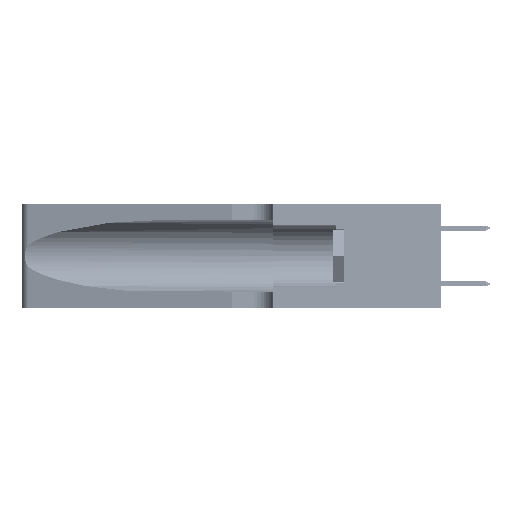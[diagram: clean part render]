
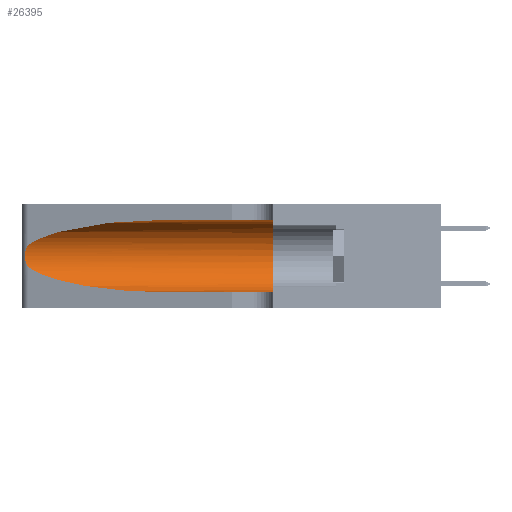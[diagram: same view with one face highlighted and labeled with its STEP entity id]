
A CAD part, left-side view. The second image highlights one B-rep face of the part: STEP entity #26395.
In plain terms, the highlighted cylindrical face has radius 3.308 mm (diameter 6.617 mm), a partial arc.
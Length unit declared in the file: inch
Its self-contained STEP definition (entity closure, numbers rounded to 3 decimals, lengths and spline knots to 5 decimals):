
#160 = CARTESIAN_POINT ( 'NONE',  ( 0.26075, 1.23896, 0.19203 ) ) ;
#484 = CARTESIAN_POINT ( 'NONE',  ( 0.25787, 1.23484, 0.2124 ) ) ;
#584 = VERTEX_POINT ( 'NONE', #38833 ) ;
#1126 = AXIS2_PLACEMENT_3D ( 'NONE', #7412, #33444, #25333 ) ;
#3918 = CARTESIAN_POINT ( 'NONE',  ( 0.25639, 1.23184, 0.21858 ) ) ;
#4160 = CARTESIAN_POINT ( 'NONE',  ( 0.25487, 1.22718, 0.22369 ) ) ;
#6103 = CYLINDRICAL_SURFACE ( 'NONE', #1126, 0.13025 ) ;
#6865 = DIRECTION ( 'NONE',  ( 0., 1., 0. ) ) ;
#7412 = CARTESIAN_POINT ( 'NONE',  ( 0.1305, 1.61858, 0.185 ) ) ;
#7413 = CIRCLE ( 'NONE', #36605, 0.13025 ) ;
#7714 = CARTESIAN_POINT ( 'NONE',  ( 0.18966, 0.96281, 0.31525 ) ) ;
#7722 = EDGE_CURVE ( 'NONE', #584, #17332, #21143, .T. ) ;
#8192 = CARTESIAN_POINT ( 'NONE',  ( 0.1305, 0.72297, 0.31525 ) ) ;
#9548 =( BOUNDED_CURVE ( )  B_SPLINE_CURVE ( 3, ( #43768, #21286, #43301, #39689 ),
 .UNSPECIFIED., .F., .F. ) 
 B_SPLINE_CURVE_WITH_KNOTS ( ( 4, 4 ),
 ( 3.44316, 4.71239 ),
 .UNSPECIFIED. ) 
 CURVE ( )  GEOMETRIC_REPRESENTATION_ITEM ( )  RATIONAL_B_SPLINE_CURVE ( ( 1., 0.87, 0.87, 1. ) ) 
 REPRESENTATION_ITEM ( '' )  );
#9904 = ORIENTED_EDGE ( 'NONE', *, *, #37767, .F. ) ;
#10907 = CARTESIAN_POINT ( 'NONE',  ( 0.25487, 1.22718, 0.14631 ) ) ;
#11216 = EDGE_CURVE ( 'NONE', #584, #25599, #27756, .T. ) ;
#14058 = CARTESIAN_POINT ( 'NONE',  ( 0.1305, 0.72297, 0.05475 ) ) ;
#14663 = ORIENTED_EDGE ( 'NONE', *, *, #36553, .T. ) ;
#15286 = CARTESIAN_POINT ( 'NONE',  ( 0.25487, 1.22718, 0.22369 ) ) ;
#15588 = ORIENTED_EDGE ( 'NONE', *, *, #11216, .T. ) ;
#17234 = EDGE_CURVE ( 'NONE', #25599, #41926, #20280, .T. ) ;
#17332 = VERTEX_POINT ( 'NONE', #23597 ) ;
#20280 = B_SPLINE_CURVE_WITH_KNOTS ( 'NONE', 3,
 ( #15286, #22461, #3918, #484, #44805, #48227, #160, #37453, #22783, #25884, #22613, #26208, #33673, #10907 ),
 .UNSPECIFIED., .F., .F.,
 ( 4, 2, 2, 2, 2, 2, 4 ),
 ( 0., 0.00027, 0.00053, 0.00107, 0.0016, 0.00187, 0.00214 ),
 .UNSPECIFIED. ) ;
#21143 = LINE ( 'NONE', #32674, #31049 ) ;
#21286 = CARTESIAN_POINT ( 'NONE',  ( 0.2373, 1.15595, 0.08982 ) ) ;
#22092 = CARTESIAN_POINT ( 'NONE',  ( 0.1305, 1.61858, 0.05475 ) ) ;
#22461 = CARTESIAN_POINT ( 'NONE',  ( 0.25555, 1.22994, 0.2215 ) ) ;
#22613 = CARTESIAN_POINT ( 'NONE',  ( 0.25789, 1.23486, 0.15765 ) ) ;
#22783 = CARTESIAN_POINT ( 'NONE',  ( 0.26017, 1.23833, 0.17102 ) ) ;
#23597 = CARTESIAN_POINT ( 'NONE',  ( 0.1305, 0.35, 0.31525 ) ) ;
#24653 = FACE_OUTER_BOUND ( 'NONE', #31269, .T. ) ;
#25333 = DIRECTION ( 'NONE',  ( 0., 0., -1. ) ) ;
#25599 = VERTEX_POINT ( 'NONE', #31252 ) ;
#25884 = CARTESIAN_POINT ( 'NONE',  ( 0.25856, 1.23593, 0.16098 ) ) ;
#26208 = CARTESIAN_POINT ( 'NONE',  ( 0.25639, 1.23186, 0.15144 ) ) ;
#26395 = ADVANCED_FACE ( 'NONE', ( #24653 ), #6103, .F. ) ;
#27756 =( BOUNDED_CURVE ( )  B_SPLINE_CURVE ( 3, ( #8192, #7714, #41251, #4160 ),
 .UNSPECIFIED., .F., .F. ) 
 B_SPLINE_CURVE_WITH_KNOTS ( ( 4, 4 ),
 ( 1.5708, 2.84003 ),
 .UNSPECIFIED. ) 
 CURVE ( )  GEOMETRIC_REPRESENTATION_ITEM ( )  RATIONAL_B_SPLINE_CURVE ( ( 1., 0.87, 0.87, 1. ) ) 
 REPRESENTATION_ITEM ( '' )  );
#29281 = DIRECTION ( 'NONE',  ( 0., -1., 0. ) ) ;
#29341 = VERTEX_POINT ( 'NONE', #38858 ) ;
#29375 = VERTEX_POINT ( 'NONE', #14058 ) ;
#31049 = VECTOR ( 'NONE', #47052, 39.37008 ) ;
#31252 = CARTESIAN_POINT ( 'NONE',  ( 0.25487, 1.22718, 0.22369 ) ) ;
#31269 = EDGE_LOOP ( 'NONE', ( #15588, #44479, #36143, #14663, #9904, #44115 ) ) ;
#32674 = CARTESIAN_POINT ( 'NONE',  ( 0.1305, 1.61858, 0.31525 ) ) ;
#33444 = DIRECTION ( 'NONE',  ( 0., -1., 0. ) ) ;
#33673 = CARTESIAN_POINT ( 'NONE',  ( 0.25555, 1.22993, 0.14849 ) ) ;
#35210 = EDGE_CURVE ( 'NONE', #41926, #29375, #9548, .T. ) ;
#36143 = ORIENTED_EDGE ( 'NONE', *, *, #35210, .T. ) ;
#36553 = EDGE_CURVE ( 'NONE', #29375, #29341, #36727, .T. ) ;
#36605 = AXIS2_PLACEMENT_3D ( 'NONE', #48054, #6865, #43981 ) ;
#36727 = LINE ( 'NONE', #22092, #43153 ) ;
#37453 = CARTESIAN_POINT ( 'NONE',  ( 0.26075, 1.23896, 0.178 ) ) ;
#37767 = EDGE_CURVE ( 'NONE', #17332, #29341, #7413, .T. ) ;
#38833 = CARTESIAN_POINT ( 'NONE',  ( 0.1305, 0.72297, 0.31525 ) ) ;
#38858 = CARTESIAN_POINT ( 'NONE',  ( 0.1305, 0.35, 0.05475 ) ) ;
#39689 = CARTESIAN_POINT ( 'NONE',  ( 0.1305, 0.72297, 0.05475 ) ) ;
#41251 = CARTESIAN_POINT ( 'NONE',  ( 0.2373, 1.15595, 0.28018 ) ) ;
#41926 = VERTEX_POINT ( 'NONE', #45478 ) ;
#43153 = VECTOR ( 'NONE', #29281, 39.37008 ) ;
#43301 = CARTESIAN_POINT ( 'NONE',  ( 0.18966, 0.96281, 0.05475 ) ) ;
#43768 = CARTESIAN_POINT ( 'NONE',  ( 0.25487, 1.22718, 0.14631 ) ) ;
#43981 = DIRECTION ( 'NONE',  ( 0., 0., 1. ) ) ;
#44115 = ORIENTED_EDGE ( 'NONE', *, *, #7722, .F. ) ;
#44479 = ORIENTED_EDGE ( 'NONE', *, *, #17234, .T. ) ;
#44805 = CARTESIAN_POINT ( 'NONE',  ( 0.25854, 1.2359, 0.20912 ) ) ;
#45478 = CARTESIAN_POINT ( 'NONE',  ( 0.25487, 1.22718, 0.14631 ) ) ;
#47052 = DIRECTION ( 'NONE',  ( 0., -1., 0. ) ) ;
#48054 = CARTESIAN_POINT ( 'NONE',  ( 0.1305, 0.35, 0.185 ) ) ;
#48227 = CARTESIAN_POINT ( 'NONE',  ( 0.26018, 1.23835, 0.19895 ) ) ;
